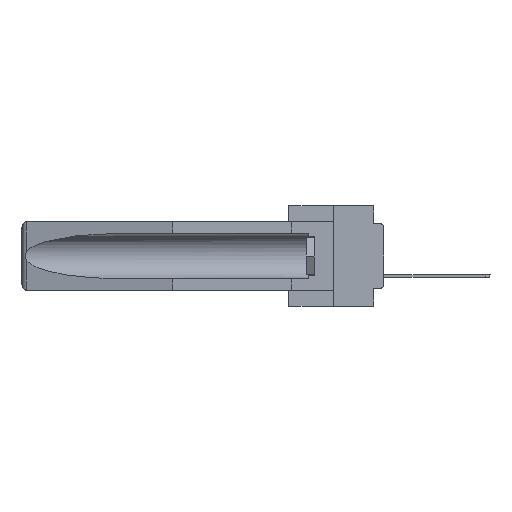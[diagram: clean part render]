
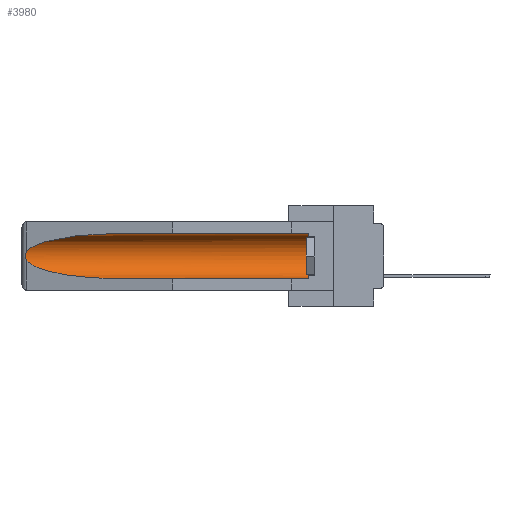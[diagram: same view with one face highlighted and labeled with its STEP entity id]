
A CAD part, left-side view. The second image highlights one B-rep face of the part: STEP entity #3980.
In plain terms, the highlighted cylindrical face has radius 2.857 mm (diameter 5.715 mm), a partial arc.
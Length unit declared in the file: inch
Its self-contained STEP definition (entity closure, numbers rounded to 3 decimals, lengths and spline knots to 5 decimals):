
#564 = EDGE_CURVE ( 'NONE', #5189, #16689, #24234, .T. ) ;
#1391 = AXIS2_PLACEMENT_3D ( 'NONE', #8189, #6467, #6041 ) ;
#2522 = VERTEX_POINT ( 'NONE', #24719 ) ;
#2607 = DIRECTION ( 'NONE',  ( 0., 1., 0. ) ) ;
#2862 = CARTESIAN_POINT ( 'NONE',  ( 0.155, 1.07973, -0.284 ) ) ;
#3441 = CARTESIAN_POINT ( 'NONE',  ( 0.26654, 1.53092, -0.15636 ) ) ;
#3489 = CARTESIAN_POINT ( 'NONE',  ( 0.26537, 1.52718, -0.19328 ) ) ;
#3670 = DIRECTION ( 'NONE',  ( 0., 1., 0. ) ) ;
#3934 = DIRECTION ( 'NONE',  ( 0., -1., 0. ) ) ;
#3980 = ADVANCED_FACE ( 'NONE', ( #4056 ), #28138, .F. ) ;
#4056 = FACE_OUTER_BOUND ( 'NONE', #25546, .T. ) ;
#4539 = CARTESIAN_POINT ( 'NONE',  ( 0.26537, 1.52718, -0.19328 ) ) ;
#5189 = VERTEX_POINT ( 'NONE', #3489 ) ;
#5191 = ORIENTED_EDGE ( 'NONE', *, *, #564, .T. ) ;
#5711 = CARTESIAN_POINT ( 'NONE',  ( 0.2673, 1.53269, -0.17917 ) ) ;
#6041 = DIRECTION ( 'NONE',  ( 0., 0., 1. ) ) ;
#6467 = DIRECTION ( 'NONE',  ( 0., 1., 0. ) ) ;
#6651 = CARTESIAN_POINT ( 'NONE',  ( 0.155, 0.126, -0.284 ) ) ;
#7856 = CARTESIAN_POINT ( 'NONE',  ( 0.2675, 1.53308, -0.16763 ) ) ;
#7993 = CARTESIAN_POINT ( 'NONE',  ( 0.26655, 1.53094, -0.18657 ) ) ;
#8189 = CARTESIAN_POINT ( 'NONE',  ( 0.155, -0.30754, -0.1715 ) ) ;
#8344 = DIRECTION ( 'NONE',  ( 0., 0., 1. ) ) ;
#8839 = ORIENTED_EDGE ( 'NONE', *, *, #22950, .F. ) ;
#9730 = B_SPLINE_CURVE_WITH_KNOTS ( 'NONE', 3,
 ( #9857, #22960, #3441, #27379, #7856, #25240, #5711, #7993, #12270, #20958 ),
 .UNSPECIFIED., .F., .F.,
 ( 4, 2, 2, 2, 4 ),
 ( 0., 0.00029, 0.00058, 0.00087, 0.00117 ),
 .UNSPECIFIED. ) ;
#9857 = CARTESIAN_POINT ( 'NONE',  ( 0.26537, 1.52718, -0.14972 ) ) ;
#10358 = EDGE_CURVE ( 'NONE', #2522, #5189, #9730, .T. ) ;
#10764 = CARTESIAN_POINT ( 'NONE',  ( 0.155, 0.126, -0.059 ) ) ;
#11383 = CARTESIAN_POINT ( 'NONE',  ( 0.21114, 1.30732, -0.059 ) ) ;
#12270 = CARTESIAN_POINT ( 'NONE',  ( 0.26597, 1.5296, -0.19026 ) ) ;
#12613 = CIRCLE ( 'NONE', #18072, 0.1125 ) ;
#13241 = CARTESIAN_POINT ( 'NONE',  ( 0.25451, 1.48313, -0.24835 ) ) ;
#13446 = LINE ( 'NONE', #22132, #24068 ) ;
#13796 = CARTESIAN_POINT ( 'NONE',  ( 0.25451, 1.48313, -0.09465 ) ) ;
#15646 = CARTESIAN_POINT ( 'NONE',  ( 0.21114, 1.30732, -0.284 ) ) ;
#16689 = VERTEX_POINT ( 'NONE', #2862 ) ;
#16707 = VERTEX_POINT ( 'NONE', #6651 ) ;
#17229 = EDGE_CURVE ( 'NONE', #17752, #25654, #25319, .T. ) ;
#17752 = VERTEX_POINT ( 'NONE', #10764 ) ;
#18072 = AXIS2_PLACEMENT_3D ( 'NONE', #27722, #3934, #8344 ) ;
#18482 = ORIENTED_EDGE ( 'NONE', *, *, #22006, .T. ) ;
#19229 = CARTESIAN_POINT ( 'NONE',  ( 0.155, 1.07973, -0.059 ) ) ;
#20404 =( BOUNDED_CURVE ( )  B_SPLINE_CURVE ( 3, ( #22474, #11383, #13796, #24196 ),
 .UNSPECIFIED., .F., .F. ) 
 B_SPLINE_CURVE_WITH_KNOTS ( ( 4, 4 ),
 ( 4.71239, 6.08839 ),
 .UNSPECIFIED. ) 
 CURVE ( )  GEOMETRIC_REPRESENTATION_ITEM ( )  RATIONAL_B_SPLINE_CURVE ( ( 1., 0.848, 0.848, 1. ) ) 
 REPRESENTATION_ITEM ( '' )  );
#20958 = CARTESIAN_POINT ( 'NONE',  ( 0.26537, 1.52718, -0.19328 ) ) ;
#21097 = EDGE_CURVE ( 'NONE', #16707, #17752, #12613, .T. ) ;
#21142 = VECTOR ( 'NONE', #3670, 39.37008 ) ;
#21924 = CARTESIAN_POINT ( 'NONE',  ( 0.155, 1.07973, -0.284 ) ) ;
#22006 = EDGE_CURVE ( 'NONE', #25654, #2522, #20404, .T. ) ;
#22132 = CARTESIAN_POINT ( 'NONE',  ( 0.155, -0.30754, -0.284 ) ) ;
#22474 = CARTESIAN_POINT ( 'NONE',  ( 0.155, 1.07973, -0.059 ) ) ;
#22855 = ORIENTED_EDGE ( 'NONE', *, *, #17229, .T. ) ;
#22950 = EDGE_CURVE ( 'NONE', #16707, #16689, #13446, .T. ) ;
#22960 = CARTESIAN_POINT ( 'NONE',  ( 0.26597, 1.52961, -0.15275 ) ) ;
#23183 = CARTESIAN_POINT ( 'NONE',  ( 0.155, -0.30754, -0.059 ) ) ;
#24068 = VECTOR ( 'NONE', #2607, 39.37008 ) ;
#24196 = CARTESIAN_POINT ( 'NONE',  ( 0.26537, 1.52718, -0.14972 ) ) ;
#24234 =( BOUNDED_CURVE ( )  B_SPLINE_CURVE ( 3, ( #4539, #13241, #15646, #21924 ),
 .UNSPECIFIED., .F., .F. ) 
 B_SPLINE_CURVE_WITH_KNOTS ( ( 4, 4 ),
 ( 0.1948, 1.5708 ),
 .UNSPECIFIED. ) 
 CURVE ( )  GEOMETRIC_REPRESENTATION_ITEM ( )  RATIONAL_B_SPLINE_CURVE ( ( 1., 0.848, 0.848, 1. ) ) 
 REPRESENTATION_ITEM ( '' )  );
#24719 = CARTESIAN_POINT ( 'NONE',  ( 0.26537, 1.52718, -0.14972 ) ) ;
#25240 = CARTESIAN_POINT ( 'NONE',  ( 0.2675, 1.53308, -0.17534 ) ) ;
#25319 = LINE ( 'NONE', #23183, #21142 ) ;
#25546 = EDGE_LOOP ( 'NONE', ( #18482, #26781, #5191, #8839, #26960, #22855 ) ) ;
#25654 = VERTEX_POINT ( 'NONE', #19229 ) ;
#26781 = ORIENTED_EDGE ( 'NONE', *, *, #10358, .T. ) ;
#26960 = ORIENTED_EDGE ( 'NONE', *, *, #21097, .T. ) ;
#27379 = CARTESIAN_POINT ( 'NONE',  ( 0.2673, 1.5327, -0.16383 ) ) ;
#27722 = CARTESIAN_POINT ( 'NONE',  ( 0.155, 0.126, -0.1715 ) ) ;
#28138 = CYLINDRICAL_SURFACE ( 'NONE', #1391, 0.1125 ) ;
